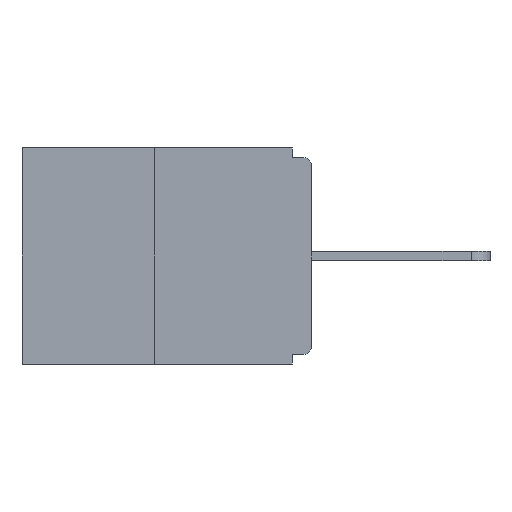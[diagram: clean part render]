
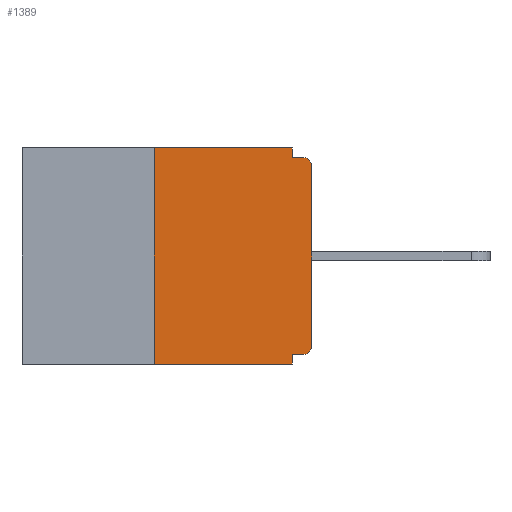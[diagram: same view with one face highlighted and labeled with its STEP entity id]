
A CAD part, left-side view. The second image highlights one B-rep face of the part: STEP entity #1389.
In plain terms, the highlighted planar face has unit normal (-1, 0, 0).
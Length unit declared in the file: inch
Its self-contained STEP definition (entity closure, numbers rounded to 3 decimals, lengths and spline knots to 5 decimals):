
#26 = ORIENTED_EDGE ( 'NONE', *, *, #2498, .T. ) ;
#304 = ORIENTED_EDGE ( 'NONE', *, *, #6096, .T. ) ;
#314 = LINE ( 'NONE', #4580, #923 ) ;
#504 = AXIS2_PLACEMENT_3D ( 'NONE', #8719, #1958, #10353 ) ;
#577 = ORIENTED_EDGE ( 'NONE', *, *, #10260, .F. ) ;
#736 = CARTESIAN_POINT ( 'NONE',  ( 0., 0., -0.015 ) ) ;
#753 = VERTEX_POINT ( 'NONE', #10395 ) ;
#923 = VECTOR ( 'NONE', #3678, 39.37008 ) ;
#925 = EDGE_CURVE ( 'NONE', #8047, #753, #9623, .T. ) ;
#1214 = VECTOR ( 'NONE', #8308, 39.37008 ) ;
#1389 = ADVANCED_FACE ( 'NONE', ( #9489 ), #5383, .F. ) ;
#1474 = CARTESIAN_POINT ( 'NONE',  ( 0., 0.46, 0. ) ) ;
#1589 = LINE ( 'NONE', #8194, #1214 ) ;
#1764 = VECTOR ( 'NONE', #10716, 39.37008 ) ;
#1833 = EDGE_CURVE ( 'NONE', #9463, #8047, #3852, .T. ) ;
#1958 = DIRECTION ( 'NONE',  ( 1., 0., 0. ) ) ;
#2498 = EDGE_CURVE ( 'NONE', #9463, #6462, #7501, .T. ) ;
#2501 = EDGE_CURVE ( 'NONE', #5030, #5746, #5883, .T. ) ;
#2559 = AXIS2_PLACEMENT_3D ( 'NONE', #8282, #7643, #3936 ) ;
#2740 = DIRECTION ( 'NONE',  ( -1., 0., 0. ) ) ;
#2795 = CARTESIAN_POINT ( 'NONE',  ( 0., 0.015, -0.313 ) ) ;
#2866 = CARTESIAN_POINT ( 'NONE',  ( 0., 0.015, -0.015 ) ) ;
#3028 = CIRCLE ( 'NONE', #4462, 0.015 ) ;
#3182 = DIRECTION ( 'NONE',  ( 0., -1., 0. ) ) ;
#3209 = DIRECTION ( 'NONE',  ( 0., -1., 0. ) ) ;
#3643 = ORIENTED_EDGE ( 'NONE', *, *, #2501, .F. ) ;
#3678 = DIRECTION ( 'NONE',  ( 0., 0., 1. ) ) ;
#3683 = VECTOR ( 'NONE', #10856, 39.37008 ) ;
#3852 = LINE ( 'NONE', #7047, #9889 ) ;
#3936 = DIRECTION ( 'NONE',  ( 0., 0., -1. ) ) ;
#4281 = CARTESIAN_POINT ( 'NONE',  ( 0., 0., -0.03 ) ) ;
#4462 = AXIS2_PLACEMENT_3D ( 'NONE', #2795, #2740, #9400 ) ;
#4485 = ORIENTED_EDGE ( 'NONE', *, *, #1833, .F. ) ;
#4580 = CARTESIAN_POINT ( 'NONE',  ( 0., 0., 0. ) ) ;
#4593 = CARTESIAN_POINT ( 'NONE',  ( 0., 0.031, -0.328 ) ) ;
#4712 = LINE ( 'NONE', #7227, #1764 ) ;
#4798 = VECTOR ( 'NONE', #3209, 39.37008 ) ;
#4807 = CARTESIAN_POINT ( 'NONE',  ( 0., 0.015, -0.328 ) ) ;
#4842 = EDGE_CURVE ( 'NONE', #5846, #7450, #1589, .T. ) ;
#5030 = VERTEX_POINT ( 'NONE', #6390 ) ;
#5142 = EDGE_CURVE ( 'NONE', #7450, #6462, #5849, .T. ) ;
#5383 = PLANE ( 'NONE',  #504 ) ;
#5616 = EDGE_CURVE ( 'NONE', #9883, #5746, #6458, .T. ) ;
#5746 = VERTEX_POINT ( 'NONE', #2866 ) ;
#5771 = DIRECTION ( 'NONE',  ( 0., -1., 0. ) ) ;
#5787 = ORIENTED_EDGE ( 'NONE', *, *, #925, .F. ) ;
#5846 = VERTEX_POINT ( 'NONE', #4807 ) ;
#5849 = LINE ( 'NONE', #10042, #3683 ) ;
#5883 = LINE ( 'NONE', #736, #10564 ) ;
#5948 = CARTESIAN_POINT ( 'NONE',  ( 0., 0.031, -0.343 ) ) ;
#6096 = EDGE_CURVE ( 'NONE', #5846, #7191, #3028, .T. ) ;
#6153 = EDGE_CURVE ( 'NONE', #7191, #9883, #314, .T. ) ;
#6228 = ORIENTED_EDGE ( 'NONE', *, *, #4842, .F. ) ;
#6390 = CARTESIAN_POINT ( 'NONE',  ( 0., 0.031, -0.015 ) ) ;
#6439 = CARTESIAN_POINT ( 'NONE',  ( 0., 0.25, 0. ) ) ;
#6458 = CIRCLE ( 'NONE', #2559, 0.015 ) ;
#6462 = VERTEX_POINT ( 'NONE', #5948 ) ;
#6579 = CARTESIAN_POINT ( 'NONE',  ( 0., 0., -0.313 ) ) ;
#7047 = CARTESIAN_POINT ( 'NONE',  ( 0., 0.25, 0. ) ) ;
#7191 = VERTEX_POINT ( 'NONE', #6579 ) ;
#7227 = CARTESIAN_POINT ( 'NONE',  ( 0., 0.031, 0. ) ) ;
#7447 = ORIENTED_EDGE ( 'NONE', *, *, #6153, .T. ) ;
#7450 = VERTEX_POINT ( 'NONE', #4593 ) ;
#7501 = LINE ( 'NONE', #9196, #4798 ) ;
#7643 = DIRECTION ( 'NONE',  ( -1., 0., 0. ) ) ;
#7950 = ORIENTED_EDGE ( 'NONE', *, *, #5142, .F. ) ;
#8042 = VECTOR ( 'NONE', #3182, 39.37008 ) ;
#8047 = VERTEX_POINT ( 'NONE', #6439 ) ;
#8194 = CARTESIAN_POINT ( 'NONE',  ( 0., 0., -0.328 ) ) ;
#8282 = CARTESIAN_POINT ( 'NONE',  ( 0., 0.015, -0.03 ) ) ;
#8308 = DIRECTION ( 'NONE',  ( 0., 1., 0. ) ) ;
#8719 = CARTESIAN_POINT ( 'NONE',  ( 0., 0.46, 0. ) ) ;
#9196 = CARTESIAN_POINT ( 'NONE',  ( 0., 0.46, -0.343 ) ) ;
#9309 = EDGE_LOOP ( 'NONE', ( #5787, #4485, #26, #7950, #6228, #304, #7447, #10114, #3643, #577 ) ) ;
#9400 = DIRECTION ( 'NONE',  ( 0., 0., -1. ) ) ;
#9463 = VERTEX_POINT ( 'NONE', #10198 ) ;
#9489 = FACE_OUTER_BOUND ( 'NONE', #9309, .T. ) ;
#9623 = LINE ( 'NONE', #1474, #8042 ) ;
#9883 = VERTEX_POINT ( 'NONE', #4281 ) ;
#9889 = VECTOR ( 'NONE', #10381, 39.37008 ) ;
#10042 = CARTESIAN_POINT ( 'NONE',  ( 0., 0.031, -0.343 ) ) ;
#10114 = ORIENTED_EDGE ( 'NONE', *, *, #5616, .T. ) ;
#10198 = CARTESIAN_POINT ( 'NONE',  ( 0., 0.25, -0.343 ) ) ;
#10260 = EDGE_CURVE ( 'NONE', #753, #5030, #4712, .T. ) ;
#10353 = DIRECTION ( 'NONE',  ( 0., 0., -1. ) ) ;
#10381 = DIRECTION ( 'NONE',  ( 0., 0., 1. ) ) ;
#10395 = CARTESIAN_POINT ( 'NONE',  ( 0., 0.031, 0. ) ) ;
#10564 = VECTOR ( 'NONE', #5771, 39.37008 ) ;
#10716 = DIRECTION ( 'NONE',  ( 0., 0., -1. ) ) ;
#10856 = DIRECTION ( 'NONE',  ( 0., 0., -1. ) ) ;
